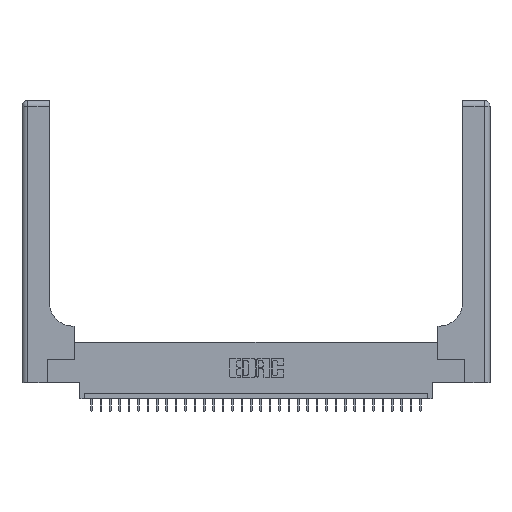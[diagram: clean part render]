
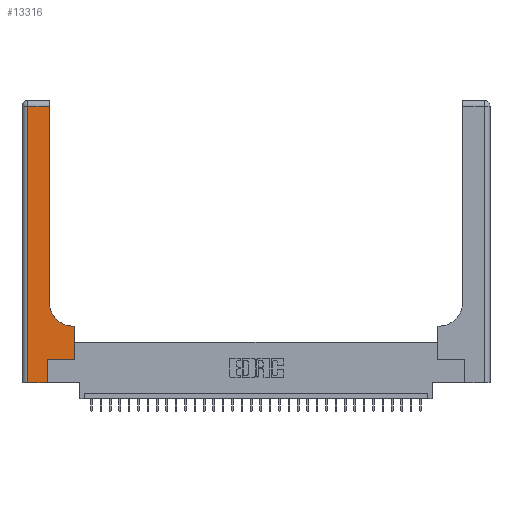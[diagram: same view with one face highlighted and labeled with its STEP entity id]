
A CAD part, top view. The second image highlights one B-rep face of the part: STEP entity #13316.
In plain terms, the highlighted planar face has unit normal (0, 0, 1).
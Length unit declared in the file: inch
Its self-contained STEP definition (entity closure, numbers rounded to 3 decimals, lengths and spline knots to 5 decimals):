
#47 = DIRECTION ( 'NONE',  ( 1., 0., 0. ) ) ;
#50 = DIRECTION ( 'NONE',  ( 0., 0., -1. ) ) ;
#75 = CIRCLE ( 'NONE', #16236, 0.25 ) ;
#224 = DIRECTION ( 'NONE',  ( 0., -1., 0. ) ) ;
#1701 = VECTOR ( 'NONE', #47, 39.37008 ) ;
#2082 = VERTEX_POINT ( 'NONE', #26041 ) ;
#2438 = VERTEX_POINT ( 'NONE', #23316 ) ;
#2860 = ORIENTED_EDGE ( 'NONE', *, *, #4923, .T. ) ;
#3081 = AXIS2_PLACEMENT_3D ( 'NONE', #23110, #50, #6304 ) ;
#3366 = VERTEX_POINT ( 'NONE', #14436 ) ;
#3480 = LINE ( 'NONE', #8703, #24473 ) ;
#4923 = EDGE_CURVE ( 'NONE', #25526, #31707, #31938, .T. ) ;
#5431 = VECTOR ( 'NONE', #7668, 39.37008 ) ;
#6304 = DIRECTION ( 'NONE',  ( -1., 0., 0. ) ) ;
#7154 = CARTESIAN_POINT ( 'NONE',  ( 0.5585, 0.25, 0.37 ) ) ;
#7668 = DIRECTION ( 'NONE',  ( 0., 1., 0. ) ) ;
#8703 = CARTESIAN_POINT ( 'NONE',  ( 0., 2.94, 0.37 ) ) ;
#8861 = CARTESIAN_POINT ( 'NONE',  ( 0.2915, 2.94, 0.37 ) ) ;
#8924 = VERTEX_POINT ( 'NONE', #15769 ) ;
#9138 = DIRECTION ( 'NONE',  ( 0., 1., 0. ) ) ;
#9177 = EDGE_CURVE ( 'NONE', #29656, #3366, #3480, .T. ) ;
#9396 = EDGE_CURVE ( 'NONE', #3366, #9612, #22960, .T. ) ;
#9612 = VERTEX_POINT ( 'NONE', #23049 ) ;
#10836 = VECTOR ( 'NONE', #24777, 39.37008 ) ;
#11094 = EDGE_CURVE ( 'NONE', #2438, #25526, #14205, .T. ) ;
#11195 = CARTESIAN_POINT ( 'NONE',  ( 0.269, 0.25, 0.37 ) ) ;
#13109 = CARTESIAN_POINT ( 'NONE',  ( 0.5415, 0.85, 0.37 ) ) ;
#13316 = ADVANCED_FACE ( 'NONE', ( #28156 ), #15389, .F. ) ;
#13431 = ORIENTED_EDGE ( 'NONE', *, *, #9177, .T. ) ;
#13815 = ORIENTED_EDGE ( 'NONE', *, *, #31237, .T. ) ;
#14205 = LINE ( 'NONE', #19075, #18105 ) ;
#14436 = CARTESIAN_POINT ( 'NONE',  ( 0.06, 2.94, 0.37 ) ) ;
#15389 = PLANE ( 'NONE',  #3081 ) ;
#15769 = CARTESIAN_POINT ( 'NONE',  ( 0.5415, 0.6, 0.37 ) ) ;
#15908 = CARTESIAN_POINT ( 'NONE',  ( 0.06, 3., 0.37 ) ) ;
#16236 = AXIS2_PLACEMENT_3D ( 'NONE', #13109, #17387, #27624 ) ;
#16453 = CARTESIAN_POINT ( 'NONE',  ( 0.269, 0.25, 0.37 ) ) ;
#17387 = DIRECTION ( 'NONE',  ( 0., 0., -1. ) ) ;
#17578 = EDGE_CURVE ( 'NONE', #31707, #2082, #32607, .T. ) ;
#18105 = VECTOR ( 'NONE', #9138, 39.37008 ) ;
#18672 = EDGE_CURVE ( 'NONE', #2082, #8924, #32537, .T. ) ;
#18971 = DIRECTION ( 'NONE',  ( 1., 0., 0. ) ) ;
#19075 = CARTESIAN_POINT ( 'NONE',  ( 0.269, 0., 0.37 ) ) ;
#19485 = CARTESIAN_POINT ( 'NONE',  ( 0.5585, 0.25, 0.37 ) ) ;
#19974 = ORIENTED_EDGE ( 'NONE', *, *, #18672, .T. ) ;
#20055 = CARTESIAN_POINT ( 'NONE',  ( 0.2915, 0.6, 0.37 ) ) ;
#22348 = LINE ( 'NONE', #24868, #5431 ) ;
#22960 = LINE ( 'NONE', #15908, #26590 ) ;
#23049 = CARTESIAN_POINT ( 'NONE',  ( 0.06, 0., 0.37 ) ) ;
#23108 = LINE ( 'NONE', #33242, #1701 ) ;
#23110 = CARTESIAN_POINT ( 'NONE',  ( 0., 3., 0.37 ) ) ;
#23238 = ORIENTED_EDGE ( 'NONE', *, *, #17578, .T. ) ;
#23316 = CARTESIAN_POINT ( 'NONE',  ( 0.269, 0., 0.37 ) ) ;
#23675 = VERTEX_POINT ( 'NONE', #25685 ) ;
#24473 = VECTOR ( 'NONE', #29048, 39.37008 ) ;
#24777 = DIRECTION ( 'NONE',  ( -1., 0., 0. ) ) ;
#24868 = CARTESIAN_POINT ( 'NONE',  ( 0.2915, 3., 0.37 ) ) ;
#25526 = VERTEX_POINT ( 'NONE', #11195 ) ;
#25685 = CARTESIAN_POINT ( 'NONE',  ( 0.2915, 0.85, 0.37 ) ) ;
#26041 = CARTESIAN_POINT ( 'NONE',  ( 0.5585, 0.6, 0.37 ) ) ;
#26590 = VECTOR ( 'NONE', #224, 39.37008 ) ;
#27285 = EDGE_LOOP ( 'NONE', ( #13815, #13431, #31316, #32558, #30496, #2860, #23238, #19974, #28624 ) ) ;
#27624 = DIRECTION ( 'NONE',  ( 1., 0., 0. ) ) ;
#27725 = VECTOR ( 'NONE', #18971, 39.37008 ) ;
#28156 = FACE_OUTER_BOUND ( 'NONE', #27285, .T. ) ;
#28624 = ORIENTED_EDGE ( 'NONE', *, *, #32074, .T. ) ;
#29048 = DIRECTION ( 'NONE',  ( -1., 0., 0. ) ) ;
#29656 = VERTEX_POINT ( 'NONE', #8861 ) ;
#29892 = DIRECTION ( 'NONE',  ( 0., 1., 0. ) ) ;
#30496 = ORIENTED_EDGE ( 'NONE', *, *, #11094, .T. ) ;
#30672 = VECTOR ( 'NONE', #29892, 39.37008 ) ;
#31237 = EDGE_CURVE ( 'NONE', #23675, #29656, #22348, .T. ) ;
#31316 = ORIENTED_EDGE ( 'NONE', *, *, #9396, .T. ) ;
#31707 = VERTEX_POINT ( 'NONE', #7154 ) ;
#31938 = LINE ( 'NONE', #16453, #27725 ) ;
#32074 = EDGE_CURVE ( 'NONE', #8924, #23675, #75, .T. ) ;
#32537 = LINE ( 'NONE', #20055, #10836 ) ;
#32558 = ORIENTED_EDGE ( 'NONE', *, *, #33032, .T. ) ;
#32607 = LINE ( 'NONE', #19485, #30672 ) ;
#33032 = EDGE_CURVE ( 'NONE', #9612, #2438, #23108, .T. ) ;
#33242 = CARTESIAN_POINT ( 'NONE',  ( 0., 0., 0.37 ) ) ;
